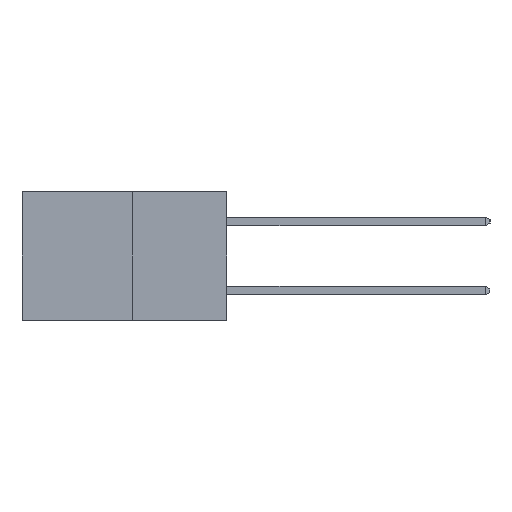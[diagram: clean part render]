
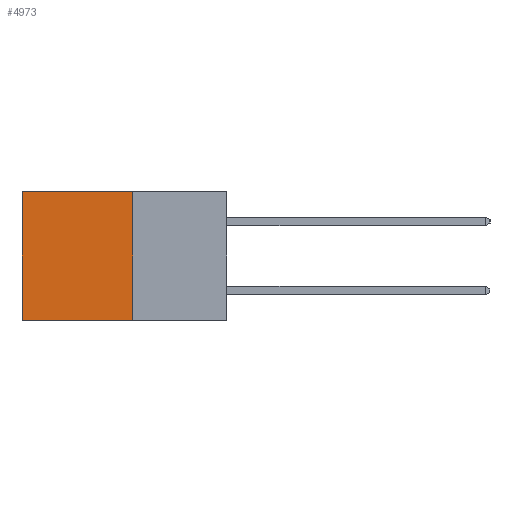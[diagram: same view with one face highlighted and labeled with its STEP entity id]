
A CAD part, left-side view. The second image highlights one B-rep face of the part: STEP entity #4973.
In plain terms, the highlighted planar face has unit normal (-1, 0, 0).
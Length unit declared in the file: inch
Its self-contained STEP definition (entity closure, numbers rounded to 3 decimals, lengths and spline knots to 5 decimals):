
#89 = VERTEX_POINT ( 'NONE', #9357 ) ;
#473 = CARTESIAN_POINT ( 'NONE',  ( 0.277, 0.27, 0. ) ) ;
#1039 = CARTESIAN_POINT ( 'NONE',  ( 0.277, 0.59, -0.37 ) ) ;
#1052 = EDGE_LOOP ( 'NONE', ( #9184, #3523, #5518, #9417 ) ) ;
#1138 = VERTEX_POINT ( 'NONE', #8914 ) ;
#2351 = LINE ( 'NONE', #9526, #8005 ) ;
#2495 = CARTESIAN_POINT ( 'NONE',  ( 0.277, 0.27, -0.37 ) ) ;
#3031 = VECTOR ( 'NONE', #9590, 39.37008 ) ;
#3140 = AXIS2_PLACEMENT_3D ( 'NONE', #5393, #5380, #5370 ) ;
#3152 = VECTOR ( 'NONE', #5751, 39.37008 ) ;
#3256 = DIRECTION ( 'NONE',  ( 0., 1., 0. ) ) ;
#3523 = ORIENTED_EDGE ( 'NONE', *, *, #7519, .F. ) ;
#4973 = ADVANCED_FACE ( 'NONE', ( #6228 ), #5404, .F. ) ;
#5370 = DIRECTION ( 'NONE',  ( 0., 0., -1. ) ) ;
#5380 = DIRECTION ( 'NONE',  ( 1., 0., 0. ) ) ;
#5393 = CARTESIAN_POINT ( 'NONE',  ( 0.277, 0.27, -0.37 ) ) ;
#5404 = PLANE ( 'NONE',  #3140 ) ;
#5481 = VECTOR ( 'NONE', #3256, 39.37008 ) ;
#5518 = ORIENTED_EDGE ( 'NONE', *, *, #6174, .F. ) ;
#5751 = DIRECTION ( 'NONE',  ( 0., 0., -1. ) ) ;
#6174 = EDGE_CURVE ( 'NONE', #8231, #8582, #2351, .T. ) ;
#6228 = FACE_OUTER_BOUND ( 'NONE', #1052, .T. ) ;
#6349 = CARTESIAN_POINT ( 'NONE',  ( 0.277, 0.27, -0.37 ) ) ;
#6856 = LINE ( 'NONE', #1039, #3152 ) ;
#7418 = LINE ( 'NONE', #2495, #5481 ) ;
#7519 = EDGE_CURVE ( 'NONE', #8582, #89, #7418, .T. ) ;
#7842 = EDGE_CURVE ( 'NONE', #1138, #89, #6856, .T. ) ;
#8005 = VECTOR ( 'NONE', #9519, 39.37008 ) ;
#8231 = VERTEX_POINT ( 'NONE', #8975 ) ;
#8582 = VERTEX_POINT ( 'NONE', #6349 ) ;
#8914 = CARTESIAN_POINT ( 'NONE',  ( 0.277, 0.59, 0. ) ) ;
#8922 = LINE ( 'NONE', #473, #3031 ) ;
#8930 = EDGE_CURVE ( 'NONE', #8231, #1138, #8922, .T. ) ;
#8975 = CARTESIAN_POINT ( 'NONE',  ( 0.277, 0.27, 0. ) ) ;
#9184 = ORIENTED_EDGE ( 'NONE', *, *, #7842, .T. ) ;
#9357 = CARTESIAN_POINT ( 'NONE',  ( 0.277, 0.59, -0.37 ) ) ;
#9417 = ORIENTED_EDGE ( 'NONE', *, *, #8930, .T. ) ;
#9519 = DIRECTION ( 'NONE',  ( 0., 0., -1. ) ) ;
#9526 = CARTESIAN_POINT ( 'NONE',  ( 0.277, 0.27, -0.37 ) ) ;
#9590 = DIRECTION ( 'NONE',  ( 0., 1., 0. ) ) ;
